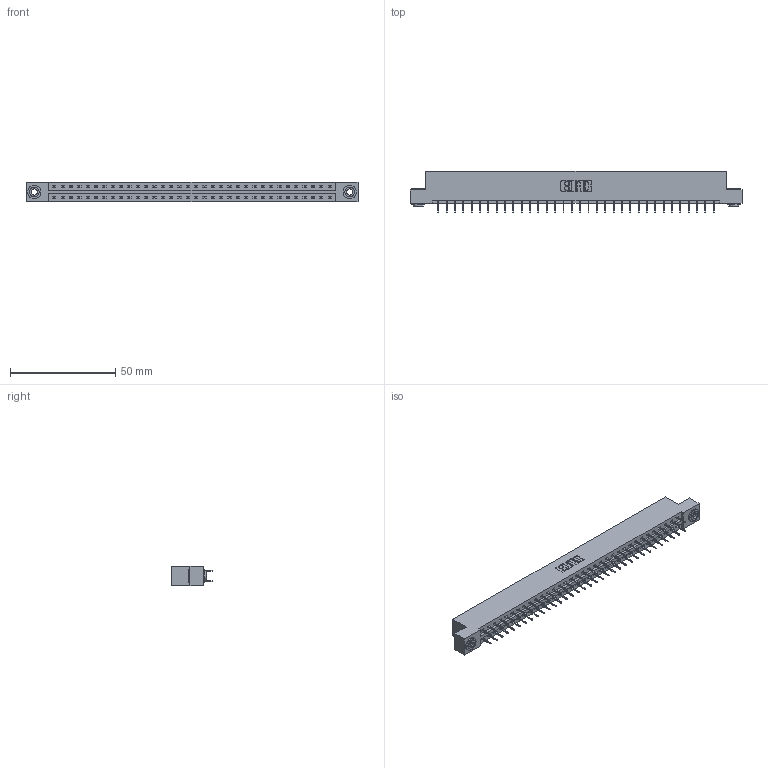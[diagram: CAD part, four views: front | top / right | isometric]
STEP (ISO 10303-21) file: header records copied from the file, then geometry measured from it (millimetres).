
FILE_DESCRIPTION (( 'STEP AP203' ), '1' );
FILE_NAME ('387-068-524-203.STEP', '2018-09-21T12:18:35', ( '' ), ( '' ), 'SwSTEP 2.0', 'SolidWorks 2016', '' );
FILE_SCHEMA (( 'CONFIG_CONTROL_DESIGN' ));
Length unit declared in the file: inch
Products named in the file (4): 337 Part_Flush Mounting Lugs - 0.156 Dia-TH; 345-292-001_345-293-124; 345-250-002_345-250-002-102; 387-068-524-203
Assembly tree (71 placements, depth 2):
  387-068-524-203
    337 Part_Flush Mounting Lugs - 0.156 Dia-TH
    345-292-001_345-293-124  x68
    345-250-002_345-250-002-102  x2
Bounding box: 157.73 x 19.69 x 9.4 mm (x, y, z)
Volume: 16433.3 mm3; surface area: 18405.8 mm2
Topology: 71 solids, 71 shells, 4096 faces, 11607 edges, 7462 vertices
Faces by surface type: plane 3072, cylinder 1016, cone 8
Entity records: 28120 total; most frequent: CARTESIAN_POINT 4717, ORIENTED_EDGE 4646, DIRECTION 4061, EDGE_CURVE 2323, VECTOR 2175, LINE 2175, VERTEX_POINT 1542, AXIS2_PLACEMENT_3D 943
